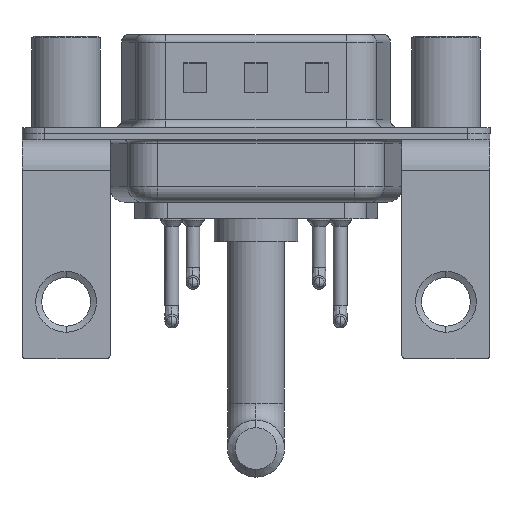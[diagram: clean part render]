
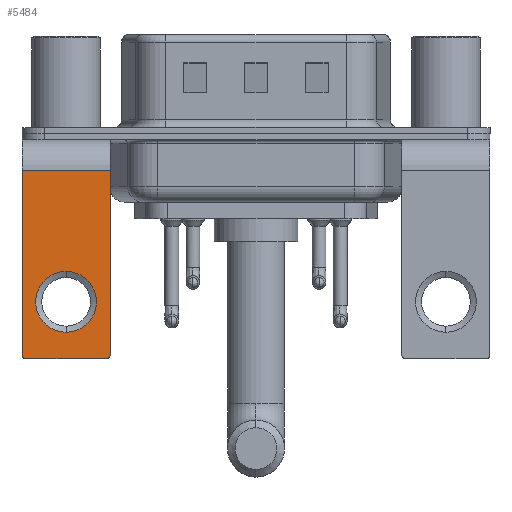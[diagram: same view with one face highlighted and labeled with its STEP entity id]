
A CAD part, front view. The second image highlights one B-rep face of the part: STEP entity #5484.
In plain terms, the highlighted planar face has unit normal (0, -1, 0).
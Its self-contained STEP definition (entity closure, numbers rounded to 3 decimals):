
#186 = LINE ( 'NONE', #18642, #15628 ) ;
#703 = CARTESIAN_POINT ( 'NONE',  ( 2.9, -6.25, -2.4 ) ) ;
#822 = DIRECTION ( 'NONE',  ( 0., 0., 1. ) ) ;
#1541 = EDGE_CURVE ( 'NONE', #6781, #7796, #12936, .T. ) ;
#1863 = VECTOR ( 'NONE', #15563, 1000. ) ;
#1902 = VECTOR ( 'NONE', #2038, 1000. ) ;
#2038 = DIRECTION ( 'NONE',  ( -1., 0., 0. ) ) ;
#2114 = CARTESIAN_POINT ( 'NONE',  ( 2.9, -6.25, -14.55 ) ) ;
#2144 = DIRECTION ( 'NONE',  ( -1., 0., 0. ) ) ;
#2391 = ORIENTED_EDGE ( 'NONE', *, *, #7549, .T. ) ;
#2517 = AXIS2_PLACEMENT_3D ( 'NONE', #4950, #10140, #6490 ) ;
#2768 = ORIENTED_EDGE ( 'NONE', *, *, #10304, .F. ) ;
#3057 = CARTESIAN_POINT ( 'NONE',  ( 2.65, -6.25, -14.8 ) ) ;
#3208 = ORIENTED_EDGE ( 'NONE', *, *, #16084, .T. ) ;
#3315 = VERTEX_POINT ( 'NONE', #2114 ) ;
#3455 = CARTESIAN_POINT ( 'NONE',  ( -2.9, -6.25, -14.55 ) ) ;
#3580 = EDGE_CURVE ( 'NONE', #14549, #12914, #10172, .T. ) ;
#3628 = CARTESIAN_POINT ( 'NONE',  ( 2.9, -6.25, -2.4 ) ) ;
#3915 = DIRECTION ( 'NONE',  ( 0., 1., 0. ) ) ;
#4950 = CARTESIAN_POINT ( 'NONE',  ( 2.9, -6.25, -2.4 ) ) ;
#5484 = ADVANCED_FACE ( 'NONE', ( #15121, #14897 ), #8490, .F. ) ;
#5515 = EDGE_CURVE ( 'NONE', #12739, #3315, #8922, .T. ) ;
#5561 = CARTESIAN_POINT ( 'NONE',  ( 2.9, -6.25, -2.4 ) ) ;
#5673 = CARTESIAN_POINT ( 'NONE',  ( 2.9, -6.25, -14.8 ) ) ;
#6326 = ORIENTED_EDGE ( 'NONE', *, *, #3580, .T. ) ;
#6490 = DIRECTION ( 'NONE',  ( 0., 0., 1. ) ) ;
#6634 = CIRCLE ( 'NONE', #11223, 0.25 ) ;
#6781 = VERTEX_POINT ( 'NONE', #16237 ) ;
#6862 = EDGE_LOOP ( 'NONE', ( #3208, #6326, #2768, #19310, #10336, #2391 ) ) ;
#6992 = EDGE_LOOP ( 'NONE', ( #15269, #17428 ) ) ;
#7222 = CARTESIAN_POINT ( 'NONE',  ( 0., -6.25, -11.07 ) ) ;
#7358 = DIRECTION ( 'NONE',  ( 0., 0., 1. ) ) ;
#7549 = EDGE_CURVE ( 'NONE', #12739, #14083, #8677, .T. ) ;
#7588 = CIRCLE ( 'NONE', #13931, 2. ) ;
#7796 = VERTEX_POINT ( 'NONE', #16729 ) ;
#8490 = PLANE ( 'NONE',  #2517 ) ;
#8677 = LINE ( 'NONE', #5561, #1902 ) ;
#8901 = CARTESIAN_POINT ( 'NONE',  ( 0., -6.25, -11.07 ) ) ;
#8922 = LINE ( 'NONE', #3628, #1863 ) ;
#10120 = AXIS2_PLACEMENT_3D ( 'NONE', #7222, #3915, #21042 ) ;
#10140 = DIRECTION ( 'NONE',  ( 0., 1., 0. ) ) ;
#10172 = CIRCLE ( 'NONE', #13711, 0.25 ) ;
#10271 = EDGE_CURVE ( 'NONE', #17585, #3315, #6634, .T. ) ;
#10304 = EDGE_CURVE ( 'NONE', #17585, #12914, #10535, .T. ) ;
#10336 = ORIENTED_EDGE ( 'NONE', *, *, #5515, .F. ) ;
#10535 = LINE ( 'NONE', #5673, #18987 ) ;
#11159 = CARTESIAN_POINT ( 'NONE',  ( -2.65, -6.25, -14.55 ) ) ;
#11223 = AXIS2_PLACEMENT_3D ( 'NONE', #18838, #15753, #822 ) ;
#12218 = DIRECTION ( 'NONE',  ( 0., 1., 0. ) ) ;
#12739 = VERTEX_POINT ( 'NONE', #703 ) ;
#12914 = VERTEX_POINT ( 'NONE', #14401 ) ;
#12936 = CIRCLE ( 'NONE', #10120, 2. ) ;
#13711 = AXIS2_PLACEMENT_3D ( 'NONE', #11159, #14800, #15256 ) ;
#13931 = AXIS2_PLACEMENT_3D ( 'NONE', #8901, #12218, #7358 ) ;
#14083 = VERTEX_POINT ( 'NONE', #16556 ) ;
#14401 = CARTESIAN_POINT ( 'NONE',  ( -2.65, -6.25, -14.8 ) ) ;
#14549 = VERTEX_POINT ( 'NONE', #3455 ) ;
#14800 = DIRECTION ( 'NONE',  ( 0., -1., 0. ) ) ;
#14897 = FACE_OUTER_BOUND ( 'NONE', #6862, .T. ) ;
#15121 = FACE_BOUND ( 'NONE', #6992, .T. ) ;
#15256 = DIRECTION ( 'NONE',  ( 0., 0., 1. ) ) ;
#15269 = ORIENTED_EDGE ( 'NONE', *, *, #19070, .T. ) ;
#15563 = DIRECTION ( 'NONE',  ( 0., 0., -1. ) ) ;
#15628 = VECTOR ( 'NONE', #17411, 1000. ) ;
#15753 = DIRECTION ( 'NONE',  ( 0., -1., 0. ) ) ;
#16084 = EDGE_CURVE ( 'NONE', #14083, #14549, #186, .T. ) ;
#16237 = CARTESIAN_POINT ( 'NONE',  ( 0., -6.25, -9.07 ) ) ;
#16556 = CARTESIAN_POINT ( 'NONE',  ( -2.9, -6.25, -2.4 ) ) ;
#16729 = CARTESIAN_POINT ( 'NONE',  ( 0., -6.25, -13.07 ) ) ;
#17411 = DIRECTION ( 'NONE',  ( 0., 0., -1. ) ) ;
#17428 = ORIENTED_EDGE ( 'NONE', *, *, #1541, .T. ) ;
#17585 = VERTEX_POINT ( 'NONE', #3057 ) ;
#18642 = CARTESIAN_POINT ( 'NONE',  ( -2.9, -6.25, -2.4 ) ) ;
#18838 = CARTESIAN_POINT ( 'NONE',  ( 2.65, -6.25, -14.55 ) ) ;
#18987 = VECTOR ( 'NONE', #2144, 1000. ) ;
#19070 = EDGE_CURVE ( 'NONE', #7796, #6781, #7588, .T. ) ;
#19310 = ORIENTED_EDGE ( 'NONE', *, *, #10271, .T. ) ;
#21042 = DIRECTION ( 'NONE',  ( 0., 0., 1. ) ) ;
